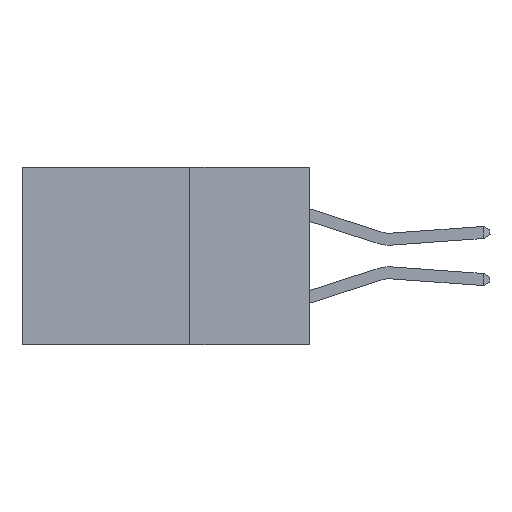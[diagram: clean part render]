
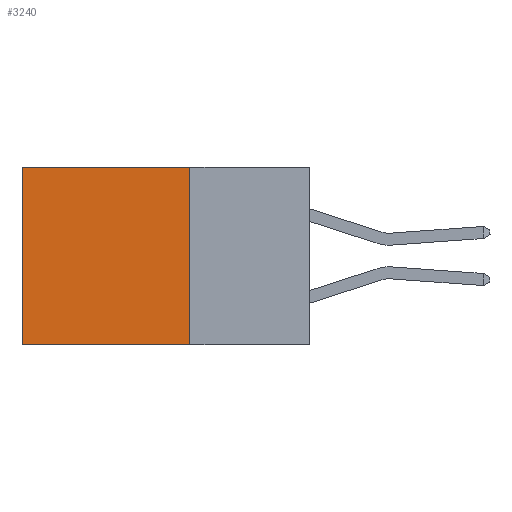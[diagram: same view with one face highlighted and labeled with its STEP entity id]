
A CAD part, left-side view. The second image highlights one B-rep face of the part: STEP entity #3240.
In plain terms, the highlighted planar face has unit normal (-1, 0, 0).
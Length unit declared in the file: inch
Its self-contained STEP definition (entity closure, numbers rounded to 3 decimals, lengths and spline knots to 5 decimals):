
#78 = CARTESIAN_POINT ( 'NONE',  ( 0.298, 0.6, 0. ) ) ;
#133 = DIRECTION ( 'NONE',  ( 0., 0., -1. ) ) ;
#496 = ORIENTED_EDGE ( 'NONE', *, *, #2648, .F. ) ;
#735 = DIRECTION ( 'NONE',  ( 0., 1., 0. ) ) ;
#1580 = CARTESIAN_POINT ( 'NONE',  ( 0.298, 0.25, -0.37 ) ) ;
#1617 = FACE_OUTER_BOUND ( 'NONE', #17739, .T. ) ;
#1918 = EDGE_CURVE ( 'NONE', #5943, #15178, #9829, .T. ) ;
#2061 = EDGE_CURVE ( 'NONE', #14206, #13712, #13839, .T. ) ;
#2643 = CARTESIAN_POINT ( 'NONE',  ( 0.298, 0.6, -0.37 ) ) ;
#2648 = EDGE_CURVE ( 'NONE', #13712, #15178, #9363, .T. ) ;
#2918 = DIRECTION ( 'NONE',  ( 0., 1., 0. ) ) ;
#3121 = CARTESIAN_POINT ( 'NONE',  ( 0.298, 0.6, 0. ) ) ;
#3240 = ADVANCED_FACE ( 'NONE', ( #1617 ), #4169, .F. ) ;
#4043 = CARTESIAN_POINT ( 'NONE',  ( 0.298, 0.25, 0. ) ) ;
#4169 = PLANE ( 'NONE',  #10533 ) ;
#5943 = VERTEX_POINT ( 'NONE', #3121 ) ;
#8438 = DIRECTION ( 'NONE',  ( 1., 0., 0. ) ) ;
#8550 = CARTESIAN_POINT ( 'NONE',  ( 0.298, 0.25, -0.37 ) ) ;
#9363 = LINE ( 'NONE', #1580, #14493 ) ;
#9773 = EDGE_CURVE ( 'NONE', #14206, #5943, #13675, .T. ) ;
#9829 = LINE ( 'NONE', #78, #15862 ) ;
#10110 = VECTOR ( 'NONE', #735, 39.37008 ) ;
#10261 = VECTOR ( 'NONE', #14901, 39.37008 ) ;
#10533 = AXIS2_PLACEMENT_3D ( 'NONE', #4043, #8438, #11350 ) ;
#10579 = ORIENTED_EDGE ( 'NONE', *, *, #9773, .T. ) ;
#10643 = ORIENTED_EDGE ( 'NONE', *, *, #1918, .T. ) ;
#10664 = CARTESIAN_POINT ( 'NONE',  ( 0.298, 0.25, 0. ) ) ;
#11350 = DIRECTION ( 'NONE',  ( 0., 0., -1. ) ) ;
#13675 = LINE ( 'NONE', #17797, #10110 ) ;
#13712 = VERTEX_POINT ( 'NONE', #8550 ) ;
#13839 = LINE ( 'NONE', #16330, #10261 ) ;
#14206 = VERTEX_POINT ( 'NONE', #10664 ) ;
#14493 = VECTOR ( 'NONE', #2918, 39.37008 ) ;
#14901 = DIRECTION ( 'NONE',  ( 0., 0., -1. ) ) ;
#15178 = VERTEX_POINT ( 'NONE', #2643 ) ;
#15862 = VECTOR ( 'NONE', #133, 39.37008 ) ;
#16330 = CARTESIAN_POINT ( 'NONE',  ( 0.298, 0.25, 0. ) ) ;
#17293 = ORIENTED_EDGE ( 'NONE', *, *, #2061, .F. ) ;
#17739 = EDGE_LOOP ( 'NONE', ( #10643, #496, #17293, #10579 ) ) ;
#17797 = CARTESIAN_POINT ( 'NONE',  ( 0.298, 0.25, 0. ) ) ;
